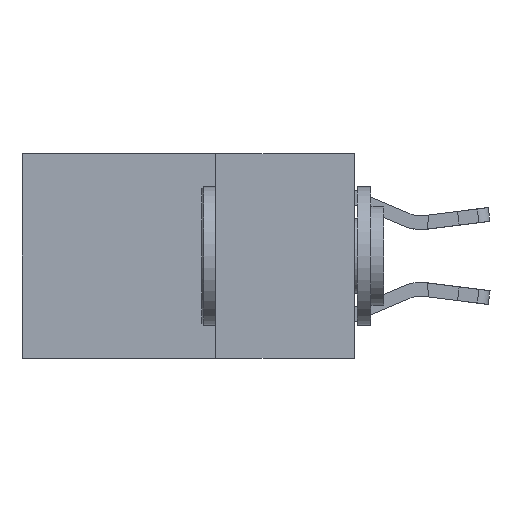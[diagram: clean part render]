
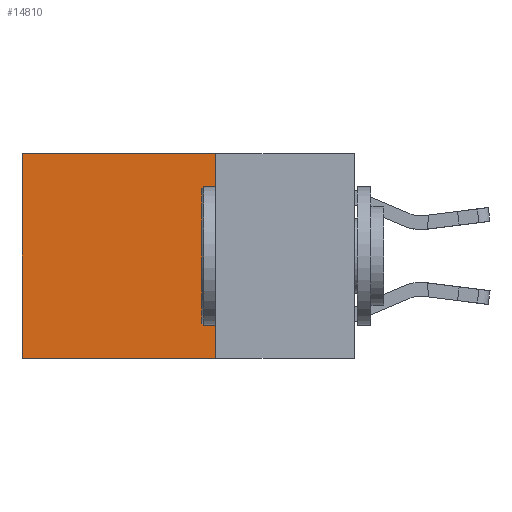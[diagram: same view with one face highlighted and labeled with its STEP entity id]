
A CAD part, left-side view. The second image highlights one B-rep face of the part: STEP entity #14810.
In plain terms, the highlighted planar face has unit normal (-1, 0, 0).
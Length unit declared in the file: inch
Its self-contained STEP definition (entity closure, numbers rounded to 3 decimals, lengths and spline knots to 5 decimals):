
#399 = VERTEX_POINT ( 'NONE', #18136 ) ;
#693 = VECTOR ( 'NONE', #6381, 39.37008 ) ;
#1138 = LINE ( 'NONE', #11808, #7673 ) ;
#1985 = EDGE_CURVE ( 'NONE', #399, #4416, #2044, .T. ) ;
#2044 = LINE ( 'NONE', #11552, #16883 ) ;
#2055 = EDGE_CURVE ( 'NONE', #4941, #4073, #20234, .T. ) ;
#3530 = EDGE_CURVE ( 'NONE', #4941, #399, #8830, .T. ) ;
#3923 = AXIS2_PLACEMENT_3D ( 'NONE', #4425, #4362, #4288 ) ;
#4073 = VERTEX_POINT ( 'NONE', #16208 ) ;
#4120 = CARTESIAN_POINT ( 'NONE',  ( 0.2625, 0.25, 0. ) ) ;
#4182 = DIRECTION ( 'NONE',  ( 0., 1., 0. ) ) ;
#4288 = DIRECTION ( 'NONE',  ( 0., 0., -1. ) ) ;
#4362 = DIRECTION ( 'NONE',  ( 1., 0., 0. ) ) ;
#4416 = VERTEX_POINT ( 'NONE', #18555 ) ;
#4425 = CARTESIAN_POINT ( 'NONE',  ( 0.2625, 0.25, 0. ) ) ;
#4941 = VERTEX_POINT ( 'NONE', #16014 ) ;
#5996 = PLANE ( 'NONE',  #3923 ) ;
#6381 = DIRECTION ( 'NONE',  ( 0., 0., -1. ) ) ;
#6617 = DIRECTION ( 'NONE',  ( 0., 1., 0. ) ) ;
#7673 = VECTOR ( 'NONE', #6617, 39.37008 ) ;
#7987 = ORIENTED_EDGE ( 'NONE', *, *, #3530, .T. ) ;
#8095 = CARTESIAN_POINT ( 'NONE',  ( 0.2625, 0.25, 0. ) ) ;
#8830 = LINE ( 'NONE', #4120, #15741 ) ;
#10275 = ORIENTED_EDGE ( 'NONE', *, *, #2055, .F. ) ;
#11552 = CARTESIAN_POINT ( 'NONE',  ( 0.2625, 0.6, 0. ) ) ;
#11592 = ORIENTED_EDGE ( 'NONE', *, *, #15829, .F. ) ;
#11808 = CARTESIAN_POINT ( 'NONE',  ( 0.2625, 0.25, -0.37 ) ) ;
#12916 = ORIENTED_EDGE ( 'NONE', *, *, #1985, .T. ) ;
#14810 = ADVANCED_FACE ( 'NONE', ( #20720 ), #5996, .F. ) ;
#15741 = VECTOR ( 'NONE', #4182, 39.37008 ) ;
#15829 = EDGE_CURVE ( 'NONE', #4073, #4416, #1138, .T. ) ;
#16014 = CARTESIAN_POINT ( 'NONE',  ( 0.2625, 0.25, 0. ) ) ;
#16208 = CARTESIAN_POINT ( 'NONE',  ( 0.2625, 0.25, -0.37 ) ) ;
#16801 = DIRECTION ( 'NONE',  ( 0., 0., -1. ) ) ;
#16883 = VECTOR ( 'NONE', #16801, 39.37008 ) ;
#18136 = CARTESIAN_POINT ( 'NONE',  ( 0.2625, 0.6, 0. ) ) ;
#18555 = CARTESIAN_POINT ( 'NONE',  ( 0.2625, 0.6, -0.37 ) ) ;
#20234 = LINE ( 'NONE', #8095, #693 ) ;
#20447 = EDGE_LOOP ( 'NONE', ( #12916, #11592, #10275, #7987 ) ) ;
#20720 = FACE_OUTER_BOUND ( 'NONE', #20447, .T. ) ;
